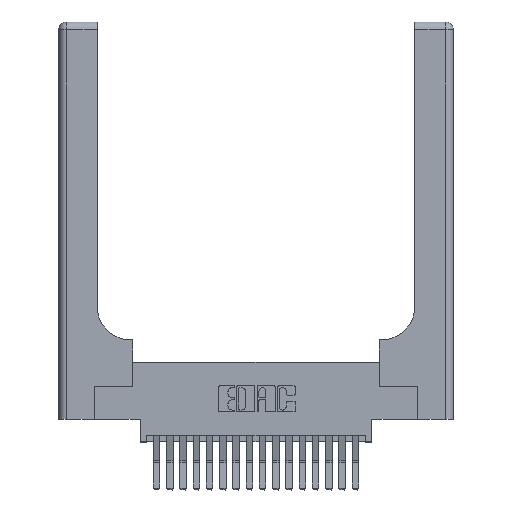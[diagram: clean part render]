
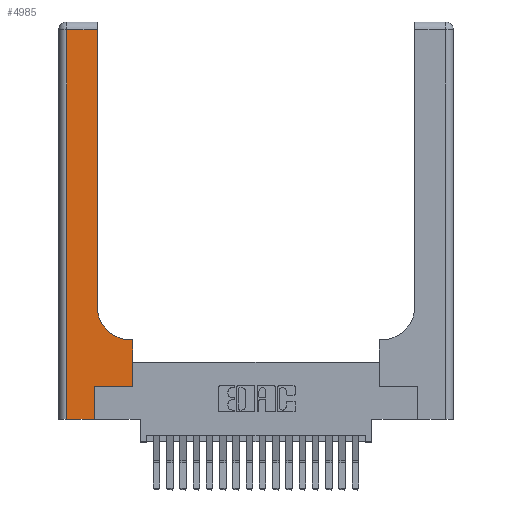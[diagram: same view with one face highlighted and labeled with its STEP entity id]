
A CAD part, top view. The second image highlights one B-rep face of the part: STEP entity #4985.
In plain terms, the highlighted planar face has unit normal (0, 0, 1).
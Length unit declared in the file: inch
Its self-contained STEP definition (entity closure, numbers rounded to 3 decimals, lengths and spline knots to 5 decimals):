
#501 = ORIENTED_EDGE ( 'NONE', *, *, #9475, .T. ) ;
#643 = DIRECTION ( 'NONE',  ( 0., -1., 0. ) ) ;
#823 = DIRECTION ( 'NONE',  ( 0., 1., 0. ) ) ;
#874 = EDGE_CURVE ( 'NONE', #8381, #21388, #14536, .T. ) ;
#1311 = CARTESIAN_POINT ( 'NONE',  ( 0.269, 0., 0.37 ) ) ;
#1771 = AXIS2_PLACEMENT_3D ( 'NONE', #14479, #4412, #16108 ) ;
#1991 = DIRECTION ( 'NONE',  ( -1., 0., 0. ) ) ;
#2225 = EDGE_CURVE ( 'NONE', #21388, #3462, #19771, .T. ) ;
#2359 = CARTESIAN_POINT ( 'NONE',  ( 0.2915, 0.6, 0.37 ) ) ;
#2390 = CARTESIAN_POINT ( 'NONE',  ( 0.06, 2.94, 0.37 ) ) ;
#2479 = CARTESIAN_POINT ( 'NONE',  ( 0.2915, 3., 0.37 ) ) ;
#3255 = EDGE_CURVE ( 'NONE', #20281, #17048, #17238, .T. ) ;
#3450 = CARTESIAN_POINT ( 'NONE',  ( 0.2915, 0.85, 0.37 ) ) ;
#3462 = VERTEX_POINT ( 'NONE', #14617 ) ;
#3683 = ORIENTED_EDGE ( 'NONE', *, *, #6557, .T. ) ;
#3689 = CARTESIAN_POINT ( 'NONE',  ( 0.269, 0.25, 0.37 ) ) ;
#3794 = CARTESIAN_POINT ( 'NONE',  ( 0.06, 0., 0.37 ) ) ;
#3880 = CARTESIAN_POINT ( 'NONE',  ( 0.2915, 2.94, 0.37 ) ) ;
#3901 = EDGE_CURVE ( 'NONE', #20031, #11741, #17974, .T. ) ;
#4079 = ORIENTED_EDGE ( 'NONE', *, *, #21465, .T. ) ;
#4412 = DIRECTION ( 'NONE',  ( 0., 0., -1. ) ) ;
#4985 = ADVANCED_FACE ( 'NONE', ( #16425 ), #10490, .F. ) ;
#5206 = DIRECTION ( 'NONE',  ( 1., 0., 0. ) ) ;
#5934 = VECTOR ( 'NONE', #6669, 39.37008 ) ;
#6149 = VECTOR ( 'NONE', #5206, 39.37008 ) ;
#6193 = LINE ( 'NONE', #1311, #18855 ) ;
#6404 = VERTEX_POINT ( 'NONE', #14669 ) ;
#6557 = EDGE_CURVE ( 'NONE', #11741, #20281, #19115, .T. ) ;
#6584 = ORIENTED_EDGE ( 'NONE', *, *, #3901, .T. ) ;
#6669 = DIRECTION ( 'NONE',  ( -1., 0., 0. ) ) ;
#6748 = DIRECTION ( 'NONE',  ( 1., 0., 0. ) ) ;
#7392 = VECTOR ( 'NONE', #643, 39.37008 ) ;
#8077 = ORIENTED_EDGE ( 'NONE', *, *, #3255, .T. ) ;
#8297 = VERTEX_POINT ( 'NONE', #17637 ) ;
#8381 = VERTEX_POINT ( 'NONE', #19455 ) ;
#8452 = CARTESIAN_POINT ( 'NONE',  ( 0., 0., 0.37 ) ) ;
#8595 = EDGE_CURVE ( 'NONE', #17048, #8297, #10047, .T. ) ;
#9067 = CARTESIAN_POINT ( 'NONE',  ( 0.06, 3., 0.37 ) ) ;
#9212 = VECTOR ( 'NONE', #823, 39.37008 ) ;
#9475 = EDGE_CURVE ( 'NONE', #3462, #6404, #13915, .T. ) ;
#10047 = LINE ( 'NONE', #8452, #18265 ) ;
#10490 = PLANE ( 'NONE',  #11426 ) ;
#11181 = ORIENTED_EDGE ( 'NONE', *, *, #874, .T. ) ;
#11319 = CARTESIAN_POINT ( 'NONE',  ( 0.5585, 0.25, 0.37 ) ) ;
#11426 = AXIS2_PLACEMENT_3D ( 'NONE', #18645, #12175, #1991 ) ;
#11741 = VERTEX_POINT ( 'NONE', #3880 ) ;
#12175 = DIRECTION ( 'NONE',  ( 0., 0., -1. ) ) ;
#12509 = ORIENTED_EDGE ( 'NONE', *, *, #17275, .T. ) ;
#12719 = EDGE_LOOP ( 'NONE', ( #6584, #3683, #8077, #18561, #4079, #11181, #15881, #501, #12509 ) ) ;
#12993 = CARTESIAN_POINT ( 'NONE',  ( 0.5585, 0.25, 0.37 ) ) ;
#13357 = CARTESIAN_POINT ( 'NONE',  ( 0., 2.94, 0.37 ) ) ;
#13404 = VECTOR ( 'NONE', #15823, 39.37008 ) ;
#13915 = LINE ( 'NONE', #2359, #13404 ) ;
#14280 = CIRCLE ( 'NONE', #1771, 0.25 ) ;
#14479 = CARTESIAN_POINT ( 'NONE',  ( 0.5415, 0.85, 0.37 ) ) ;
#14536 = LINE ( 'NONE', #3689, #6149 ) ;
#14617 = CARTESIAN_POINT ( 'NONE',  ( 0.5585, 0.6, 0.37 ) ) ;
#14669 = CARTESIAN_POINT ( 'NONE',  ( 0.5415, 0.6, 0.37 ) ) ;
#15470 = VECTOR ( 'NONE', #16277, 39.37008 ) ;
#15823 = DIRECTION ( 'NONE',  ( -1., 0., 0. ) ) ;
#15881 = ORIENTED_EDGE ( 'NONE', *, *, #2225, .T. ) ;
#16108 = DIRECTION ( 'NONE',  ( 1., 0., 0. ) ) ;
#16277 = DIRECTION ( 'NONE',  ( 0., 1., 0. ) ) ;
#16425 = FACE_OUTER_BOUND ( 'NONE', #12719, .T. ) ;
#17048 = VERTEX_POINT ( 'NONE', #3794 ) ;
#17238 = LINE ( 'NONE', #9067, #7392 ) ;
#17275 = EDGE_CURVE ( 'NONE', #6404, #20031, #14280, .T. ) ;
#17637 = CARTESIAN_POINT ( 'NONE',  ( 0.269, 0., 0.37 ) ) ;
#17966 = DIRECTION ( 'NONE',  ( 0., 1., 0. ) ) ;
#17974 = LINE ( 'NONE', #2479, #9212 ) ;
#18265 = VECTOR ( 'NONE', #6748, 39.37008 ) ;
#18561 = ORIENTED_EDGE ( 'NONE', *, *, #8595, .T. ) ;
#18645 = CARTESIAN_POINT ( 'NONE',  ( 0., 3., 0.37 ) ) ;
#18855 = VECTOR ( 'NONE', #17966, 39.37008 ) ;
#19115 = LINE ( 'NONE', #13357, #5934 ) ;
#19455 = CARTESIAN_POINT ( 'NONE',  ( 0.269, 0.25, 0.37 ) ) ;
#19771 = LINE ( 'NONE', #12993, #15470 ) ;
#20031 = VERTEX_POINT ( 'NONE', #3450 ) ;
#20281 = VERTEX_POINT ( 'NONE', #2390 ) ;
#21388 = VERTEX_POINT ( 'NONE', #11319 ) ;
#21465 = EDGE_CURVE ( 'NONE', #8297, #8381, #6193, .T. ) ;
